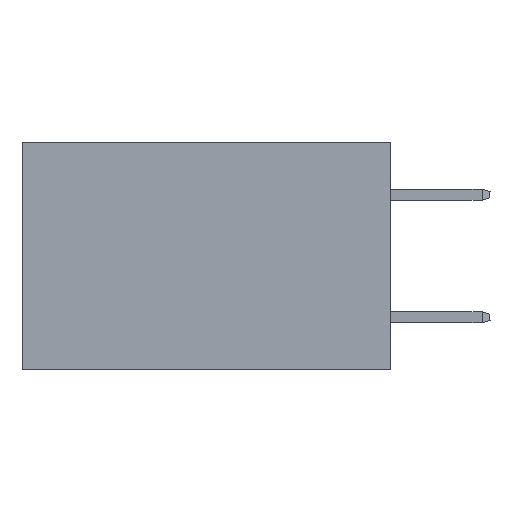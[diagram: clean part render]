
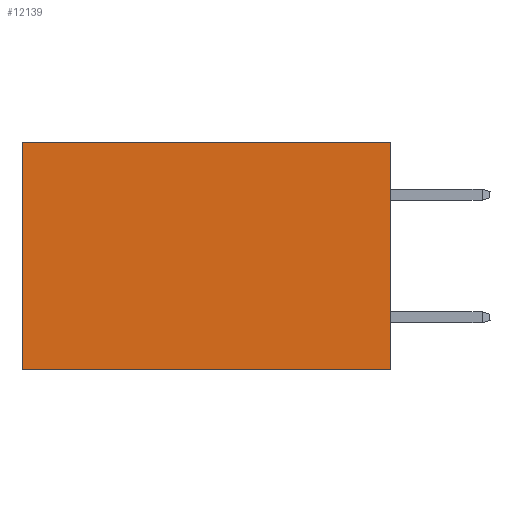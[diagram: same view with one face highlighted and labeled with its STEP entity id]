
A CAD part, left-side view. The second image highlights one B-rep face of the part: STEP entity #12139.
In plain terms, the highlighted planar face has unit normal (-1, 0, 0).
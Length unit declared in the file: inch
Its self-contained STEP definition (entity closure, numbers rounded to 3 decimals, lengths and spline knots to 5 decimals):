
#454 = VERTEX_POINT ( 'NONE', #13390 ) ;
#498 = VECTOR ( 'NONE', #10886, 39.37008 ) ;
#2632 = CARTESIAN_POINT ( 'NONE',  ( 0.2875, 0.6, 0. ) ) ;
#3149 = LINE ( 'NONE', #3214, #11968 ) ;
#3214 = CARTESIAN_POINT ( 'NONE',  ( 0.2875, 0., 0. ) ) ;
#3728 = CARTESIAN_POINT ( 'NONE',  ( 0.2875, 0., 0. ) ) ;
#3957 = LINE ( 'NONE', #2632, #21021 ) ;
#4836 = ORIENTED_EDGE ( 'NONE', *, *, #14421, .F. ) ;
#5290 = DIRECTION ( 'NONE',  ( 0., 1., 0. ) ) ;
#5458 = VERTEX_POINT ( 'NONE', #17206 ) ;
#6388 = VECTOR ( 'NONE', #5290, 39.37008 ) ;
#7097 = DIRECTION ( 'NONE',  ( 0., 0., -1. ) ) ;
#9226 = CARTESIAN_POINT ( 'NONE',  ( 0.2875, 0., 0. ) ) ;
#9602 = ORIENTED_EDGE ( 'NONE', *, *, #10661, .T. ) ;
#10661 = EDGE_CURVE ( 'NONE', #454, #19867, #3149, .T. ) ;
#10886 = DIRECTION ( 'NONE',  ( 0., 0., -1. ) ) ;
#11308 = AXIS2_PLACEMENT_3D ( 'NONE', #3728, #16713, #7097 ) ;
#11967 = ORIENTED_EDGE ( 'NONE', *, *, #17879, .T. ) ;
#11968 = VECTOR ( 'NONE', #14658, 39.37008 ) ;
#11996 = PLANE ( 'NONE',  #11308 ) ;
#12139 = ADVANCED_FACE ( 'NONE', ( #12918 ), #11996, .F. ) ;
#12456 = EDGE_LOOP ( 'NONE', ( #11967, #4836, #13700, #9602 ) ) ;
#12918 = FACE_OUTER_BOUND ( 'NONE', #12456, .T. ) ;
#13390 = CARTESIAN_POINT ( 'NONE',  ( 0.2875, 0., 0. ) ) ;
#13700 = ORIENTED_EDGE ( 'NONE', *, *, #15917, .F. ) ;
#13772 = VERTEX_POINT ( 'NONE', #14799 ) ;
#13796 = LINE ( 'NONE', #9226, #498 ) ;
#14134 = DIRECTION ( 'NONE',  ( 0., 0., -1. ) ) ;
#14421 = EDGE_CURVE ( 'NONE', #5458, #13772, #15506, .T. ) ;
#14658 = DIRECTION ( 'NONE',  ( 0., 1., 0. ) ) ;
#14799 = CARTESIAN_POINT ( 'NONE',  ( 0.2875, 0.6, -0.37 ) ) ;
#15506 = LINE ( 'NONE', #18095, #6388 ) ;
#15917 = EDGE_CURVE ( 'NONE', #454, #5458, #13796, .T. ) ;
#16713 = DIRECTION ( 'NONE',  ( 1., 0., 0. ) ) ;
#16782 = CARTESIAN_POINT ( 'NONE',  ( 0.2875, 0.6, 0. ) ) ;
#17206 = CARTESIAN_POINT ( 'NONE',  ( 0.2875, 0., -0.37 ) ) ;
#17879 = EDGE_CURVE ( 'NONE', #19867, #13772, #3957, .T. ) ;
#18095 = CARTESIAN_POINT ( 'NONE',  ( 0.2875, 0., -0.37 ) ) ;
#19867 = VERTEX_POINT ( 'NONE', #16782 ) ;
#21021 = VECTOR ( 'NONE', #14134, 39.37008 ) ;
